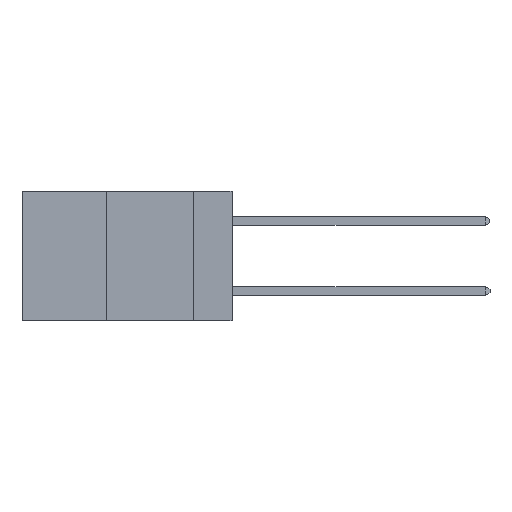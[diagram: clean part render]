
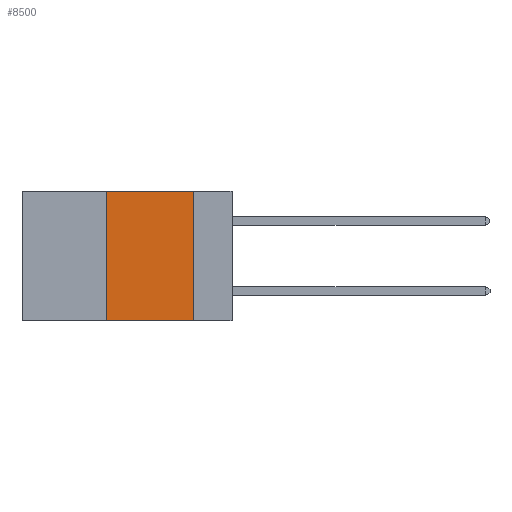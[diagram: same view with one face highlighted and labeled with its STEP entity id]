
A CAD part, left-side view. The second image highlights one B-rep face of the part: STEP entity #8500.
In plain terms, the highlighted planar face has unit normal (-1, 0, 0).
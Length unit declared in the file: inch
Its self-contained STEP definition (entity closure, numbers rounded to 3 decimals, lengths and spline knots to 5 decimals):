
#950 = EDGE_LOOP ( 'NONE', ( #20413, #12140, #16801, #21493 ) ) ;
#1079 = VECTOR ( 'NONE', #15295, 39.37008 ) ;
#1692 = LINE ( 'NONE', #9966, #1079 ) ;
#2452 = VECTOR ( 'NONE', #16050, 39.37008 ) ;
#3423 = DIRECTION ( 'NONE',  ( 0., -1., 0. ) ) ;
#4273 = PLANE ( 'NONE',  #12608 ) ;
#4315 = FACE_OUTER_BOUND ( 'NONE', #950, .T. ) ;
#5257 = VECTOR ( 'NONE', #3423, 39.37008 ) ;
#6134 = CARTESIAN_POINT ( 'NONE',  ( 0., 0.6, 0. ) ) ;
#6207 = DIRECTION ( 'NONE',  ( 0., 0., -1. ) ) ;
#8166 = LINE ( 'NONE', #14291, #2452 ) ;
#8500 = ADVANCED_FACE ( 'NONE', ( #4315 ), #4273, .F. ) ;
#9354 = VECTOR ( 'NONE', #19825, 39.37008 ) ;
#9466 = EDGE_CURVE ( 'NONE', #12114, #19214, #8166, .T. ) ;
#9966 = CARTESIAN_POINT ( 'NONE',  ( 0., 0.36, 0. ) ) ;
#10930 = CARTESIAN_POINT ( 'NONE',  ( 0., 0.36, -0.37 ) ) ;
#11280 = VERTEX_POINT ( 'NONE', #10930 ) ;
#12114 = VERTEX_POINT ( 'NONE', #20379 ) ;
#12140 = ORIENTED_EDGE ( 'NONE', *, *, #20422, .F. ) ;
#12608 = AXIS2_PLACEMENT_3D ( 'NONE', #6134, #17001, #6207 ) ;
#12686 = CARTESIAN_POINT ( 'NONE',  ( 0., 0.6, 0. ) ) ;
#13044 = EDGE_CURVE ( 'NONE', #11280, #23259, #1692, .T. ) ;
#14073 = LINE ( 'NONE', #16250, #9354 ) ;
#14291 = CARTESIAN_POINT ( 'NONE',  ( 0., 0.11, 0. ) ) ;
#15295 = DIRECTION ( 'NONE',  ( 0., 0., 1. ) ) ;
#16050 = DIRECTION ( 'NONE',  ( 0., 0., -1. ) ) ;
#16250 = CARTESIAN_POINT ( 'NONE',  ( 0., 0.6, -0.37 ) ) ;
#16801 = ORIENTED_EDGE ( 'NONE', *, *, #13044, .F. ) ;
#17001 = DIRECTION ( 'NONE',  ( 1., 0., 0. ) ) ;
#19214 = VERTEX_POINT ( 'NONE', #23444 ) ;
#19669 = LINE ( 'NONE', #12686, #5257 ) ;
#19825 = DIRECTION ( 'NONE',  ( 0., -1., 0. ) ) ;
#20379 = CARTESIAN_POINT ( 'NONE',  ( 0., 0.11, 0. ) ) ;
#20413 = ORIENTED_EDGE ( 'NONE', *, *, #9466, .F. ) ;
#20422 = EDGE_CURVE ( 'NONE', #23259, #12114, #19669, .T. ) ;
#21493 = ORIENTED_EDGE ( 'NONE', *, *, #21536, .T. ) ;
#21536 = EDGE_CURVE ( 'NONE', #11280, #19214, #14073, .T. ) ;
#23228 = CARTESIAN_POINT ( 'NONE',  ( 0., 0.36, 0. ) ) ;
#23259 = VERTEX_POINT ( 'NONE', #23228 ) ;
#23444 = CARTESIAN_POINT ( 'NONE',  ( 0., 0.11, -0.37 ) ) ;
